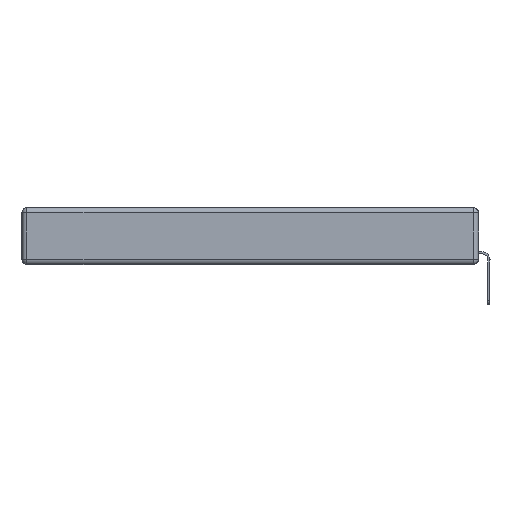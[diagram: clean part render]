
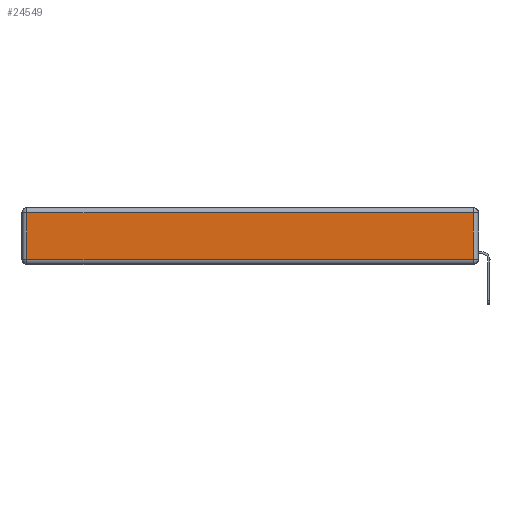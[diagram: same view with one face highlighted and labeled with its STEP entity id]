
A CAD part, left-side view. The second image highlights one B-rep face of the part: STEP entity #24549.
In plain terms, the highlighted planar face has unit normal (-1, 0, 0).
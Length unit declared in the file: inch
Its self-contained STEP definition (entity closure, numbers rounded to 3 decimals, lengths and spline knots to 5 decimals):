
#38 = CARTESIAN_POINT ( 'NONE',  ( 0., 0.03, -0.03 ) ) ;
#250 = LINE ( 'NONE', #21242, #19140 ) ;
#319 = VERTEX_POINT ( 'NONE', #2432 ) ;
#381 = LINE ( 'NONE', #6867, #23031 ) ;
#1363 = CARTESIAN_POINT ( 'NONE',  ( 0., 0., -0.343 ) ) ;
#2432 = CARTESIAN_POINT ( 'NONE',  ( 0., 2.72, -0.03 ) ) ;
#2529 = DIRECTION ( 'NONE',  ( 0., 1., 0. ) ) ;
#3175 = VECTOR ( 'NONE', #2529, 39.37008 ) ;
#5117 = ORIENTED_EDGE ( 'NONE', *, *, #5281, .T. ) ;
#5281 = EDGE_CURVE ( 'NONE', #15486, #319, #17323, .T. ) ;
#6689 = ORIENTED_EDGE ( 'NONE', *, *, #17878, .T. ) ;
#6867 = CARTESIAN_POINT ( 'NONE',  ( 0., 0., -0.313 ) ) ;
#9604 = EDGE_CURVE ( 'NONE', #27214, #15486, #250, .T. ) ;
#12062 = DIRECTION ( 'NONE',  ( 0., 0., 1. ) ) ;
#12525 = CARTESIAN_POINT ( 'NONE',  ( 0., 0.03, -0.313 ) ) ;
#12638 = ORIENTED_EDGE ( 'NONE', *, *, #21793, .T. ) ;
#13200 = EDGE_LOOP ( 'NONE', ( #6689, #17647, #5117, #12638 ) ) ;
#14313 = FACE_OUTER_BOUND ( 'NONE', #13200, .T. ) ;
#14888 = DIRECTION ( 'NONE',  ( 0., 0., 1. ) ) ;
#15486 = VERTEX_POINT ( 'NONE', #38 ) ;
#16858 = DIRECTION ( 'NONE',  ( -1., 0., 0. ) ) ;
#17231 = CARTESIAN_POINT ( 'NONE',  ( 0., 2.72, -0.313 ) ) ;
#17323 = LINE ( 'NONE', #21839, #3175 ) ;
#17647 = ORIENTED_EDGE ( 'NONE', *, *, #9604, .T. ) ;
#17878 = EDGE_CURVE ( 'NONE', #23926, #27214, #381, .T. ) ;
#19140 = VECTOR ( 'NONE', #14888, 39.37008 ) ;
#19500 = DIRECTION ( 'NONE',  ( 0., 0., -1. ) ) ;
#21223 = VECTOR ( 'NONE', #19500, 39.37008 ) ;
#21242 = CARTESIAN_POINT ( 'NONE',  ( 0., 0.03, -0.343 ) ) ;
#21756 = AXIS2_PLACEMENT_3D ( 'NONE', #1363, #16858, #12062 ) ;
#21793 = EDGE_CURVE ( 'NONE', #319, #23926, #22168, .T. ) ;
#21839 = CARTESIAN_POINT ( 'NONE',  ( 0., 2.75, -0.03 ) ) ;
#22168 = LINE ( 'NONE', #23875, #21223 ) ;
#22920 = PLANE ( 'NONE',  #21756 ) ;
#23031 = VECTOR ( 'NONE', #26041, 39.37008 ) ;
#23875 = CARTESIAN_POINT ( 'NONE',  ( 0., 2.72, -0.343 ) ) ;
#23926 = VERTEX_POINT ( 'NONE', #17231 ) ;
#24549 = ADVANCED_FACE ( 'NONE', ( #14313 ), #22920, .T. ) ;
#26041 = DIRECTION ( 'NONE',  ( 0., -1., 0. ) ) ;
#27214 = VERTEX_POINT ( 'NONE', #12525 ) ;
